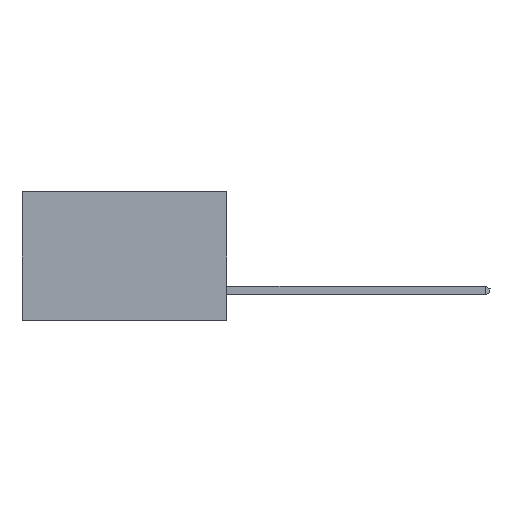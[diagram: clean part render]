
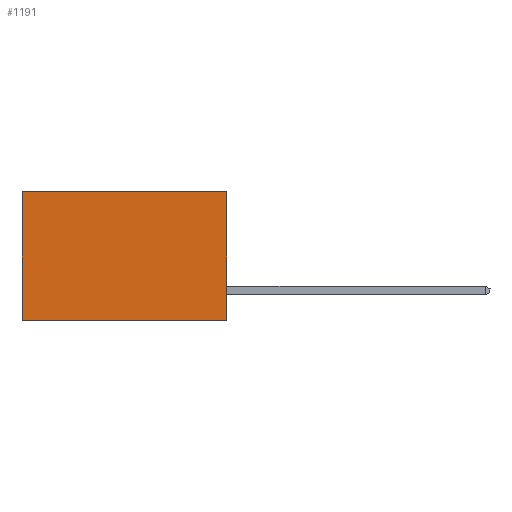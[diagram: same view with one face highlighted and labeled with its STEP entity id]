
A CAD part, left-side view. The second image highlights one B-rep face of the part: STEP entity #1191.
In plain terms, the highlighted planar face has unit normal (-1, 0, 0).
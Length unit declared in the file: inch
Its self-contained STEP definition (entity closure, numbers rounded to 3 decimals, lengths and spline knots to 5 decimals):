
#16 = VERTEX_POINT ( 'NONE', #10521 ) ;
#737 = AXIS2_PLACEMENT_3D ( 'NONE', #9844, #14226, #14124 ) ;
#978 = FACE_OUTER_BOUND ( 'NONE', #1203, .T. ) ;
#1191 = ADVANCED_FACE ( 'NONE', ( #978 ), #2404, .F. ) ;
#1203 = EDGE_LOOP ( 'NONE', ( #7157, #4905, #3338, #5833 ) ) ;
#1674 = LINE ( 'NONE', #7689, #13564 ) ;
#2404 = PLANE ( 'NONE',  #737 ) ;
#2536 = VERTEX_POINT ( 'NONE', #13157 ) ;
#3338 = ORIENTED_EDGE ( 'NONE', *, *, #13401, .F. ) ;
#3627 = CARTESIAN_POINT ( 'NONE',  ( 0.277, 0., 0. ) ) ;
#4905 = ORIENTED_EDGE ( 'NONE', *, *, #10773, .F. ) ;
#4913 = VECTOR ( 'NONE', #13413, 39.37008 ) ;
#4919 = VECTOR ( 'NONE', #10592, 39.37008 ) ;
#5046 = VERTEX_POINT ( 'NONE', #6057 ) ;
#5833 = ORIENTED_EDGE ( 'NONE', *, *, #9783, .T. ) ;
#6057 = CARTESIAN_POINT ( 'NONE',  ( 0.277, 0.59, 0. ) ) ;
#6606 = CARTESIAN_POINT ( 'NONE',  ( 0.277, 0., -0.37 ) ) ;
#7157 = ORIENTED_EDGE ( 'NONE', *, *, #14408, .T. ) ;
#7689 = CARTESIAN_POINT ( 'NONE',  ( 0.277, 0., -0.37 ) ) ;
#8127 = LINE ( 'NONE', #9041, #4913 ) ;
#8484 = LINE ( 'NONE', #3627, #4919 ) ;
#8856 = DIRECTION ( 'NONE',  ( 0., 1., 0. ) ) ;
#9041 = CARTESIAN_POINT ( 'NONE',  ( 0.277, 0.59, -0.37 ) ) ;
#9783 = EDGE_CURVE ( 'NONE', #2536, #5046, #8484, .T. ) ;
#9844 = CARTESIAN_POINT ( 'NONE',  ( 0.277, 0., -0.37 ) ) ;
#10521 = CARTESIAN_POINT ( 'NONE',  ( 0.277, 0., -0.37 ) ) ;
#10592 = DIRECTION ( 'NONE',  ( 0., 1., 0. ) ) ;
#10773 = EDGE_CURVE ( 'NONE', #16, #12516, #1674, .T. ) ;
#11474 = LINE ( 'NONE', #6606, #14263 ) ;
#12516 = VERTEX_POINT ( 'NONE', #14098 ) ;
#13157 = CARTESIAN_POINT ( 'NONE',  ( 0.277, 0., 0. ) ) ;
#13401 = EDGE_CURVE ( 'NONE', #2536, #16, #11474, .T. ) ;
#13413 = DIRECTION ( 'NONE',  ( 0., 0., -1. ) ) ;
#13564 = VECTOR ( 'NONE', #8856, 39.37008 ) ;
#14098 = CARTESIAN_POINT ( 'NONE',  ( 0.277, 0.59, -0.37 ) ) ;
#14124 = DIRECTION ( 'NONE',  ( 0., 0., -1. ) ) ;
#14226 = DIRECTION ( 'NONE',  ( 1., 0., 0. ) ) ;
#14263 = VECTOR ( 'NONE', #14347, 39.37008 ) ;
#14347 = DIRECTION ( 'NONE',  ( 0., 0., -1. ) ) ;
#14408 = EDGE_CURVE ( 'NONE', #5046, #12516, #8127, .T. ) ;
